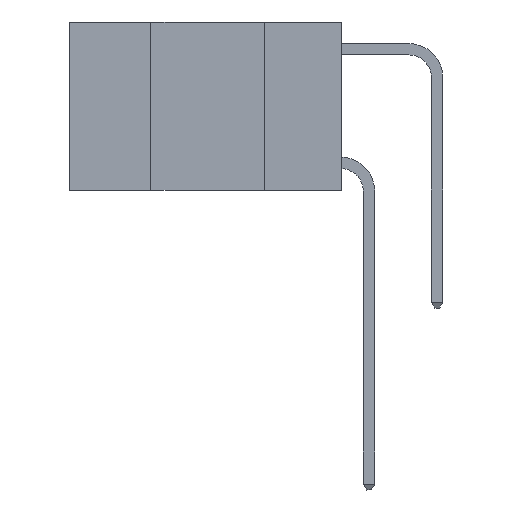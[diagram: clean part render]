
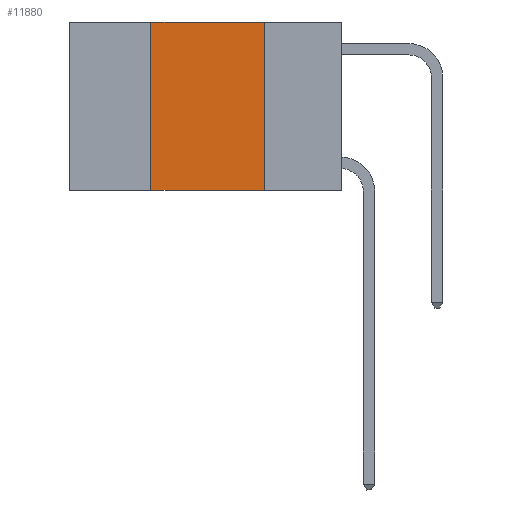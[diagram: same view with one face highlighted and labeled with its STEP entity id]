
A CAD part, left-side view. The second image highlights one B-rep face of the part: STEP entity #11880.
In plain terms, the highlighted planar face has unit normal (-1, 0, 0).
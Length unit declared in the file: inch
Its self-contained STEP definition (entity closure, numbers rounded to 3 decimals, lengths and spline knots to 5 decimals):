
#802 = EDGE_CURVE ( 'NONE', #6601, #1227, #10742, .T. ) ;
#912 = DIRECTION ( 'NONE',  ( 0., 0., -1. ) ) ;
#1227 = VERTEX_POINT ( 'NONE', #3905 ) ;
#1239 = ORIENTED_EDGE ( 'NONE', *, *, #1594, .F. ) ;
#1553 = ORIENTED_EDGE ( 'NONE', *, *, #802, .T. ) ;
#1594 = EDGE_CURVE ( 'NONE', #6982, #10939, #6923, .T. ) ;
#1706 = EDGE_CURVE ( 'NONE', #6601, #6982, #11990, .T. ) ;
#1729 = ORIENTED_EDGE ( 'NONE', *, *, #2598, .F. ) ;
#1913 = VECTOR ( 'NONE', #8259, 39.37008 ) ;
#2598 = EDGE_CURVE ( 'NONE', #10939, #1227, #4187, .T. ) ;
#2901 = DIRECTION ( 'NONE',  ( 1., 0., 0. ) ) ;
#3048 = VECTOR ( 'NONE', #9990, 39.37008 ) ;
#3314 = CARTESIAN_POINT ( 'NONE',  ( 0., 0.6, 0. ) ) ;
#3905 = CARTESIAN_POINT ( 'NONE',  ( 0., 0.17, -0.37 ) ) ;
#4187 = LINE ( 'NONE', #8219, #1913 ) ;
#4792 = PLANE ( 'NONE',  #8778 ) ;
#4825 = DIRECTION ( 'NONE',  ( 0., 0., 1. ) ) ;
#5172 = CARTESIAN_POINT ( 'NONE',  ( 0., 0.6, -0.37 ) ) ;
#5766 = CARTESIAN_POINT ( 'NONE',  ( 0., 0.6, 0. ) ) ;
#6071 = CARTESIAN_POINT ( 'NONE',  ( 0., 0.17, 0. ) ) ;
#6601 = VERTEX_POINT ( 'NONE', #10878 ) ;
#6783 = DIRECTION ( 'NONE',  ( 0., -1., 0. ) ) ;
#6886 = ORIENTED_EDGE ( 'NONE', *, *, #1706, .F. ) ;
#6923 = LINE ( 'NONE', #3314, #11094 ) ;
#6982 = VERTEX_POINT ( 'NONE', #8199 ) ;
#8199 = CARTESIAN_POINT ( 'NONE',  ( 0., 0.42, 0. ) ) ;
#8219 = CARTESIAN_POINT ( 'NONE',  ( 0., 0.17, 0. ) ) ;
#8259 = DIRECTION ( 'NONE',  ( 0., 0., -1. ) ) ;
#8262 = EDGE_LOOP ( 'NONE', ( #1729, #1239, #6886, #1553 ) ) ;
#8778 = AXIS2_PLACEMENT_3D ( 'NONE', #5766, #2901, #912 ) ;
#8901 = FACE_OUTER_BOUND ( 'NONE', #8262, .T. ) ;
#9541 = VECTOR ( 'NONE', #4825, 39.37008 ) ;
#9990 = DIRECTION ( 'NONE',  ( 0., -1., 0. ) ) ;
#10742 = LINE ( 'NONE', #5172, #3048 ) ;
#10878 = CARTESIAN_POINT ( 'NONE',  ( 0., 0.42, -0.37 ) ) ;
#10939 = VERTEX_POINT ( 'NONE', #6071 ) ;
#11094 = VECTOR ( 'NONE', #6783, 39.37008 ) ;
#11683 = CARTESIAN_POINT ( 'NONE',  ( 0., 0.42, 0. ) ) ;
#11880 = ADVANCED_FACE ( 'NONE', ( #8901 ), #4792, .F. ) ;
#11990 = LINE ( 'NONE', #11683, #9541 ) ;
